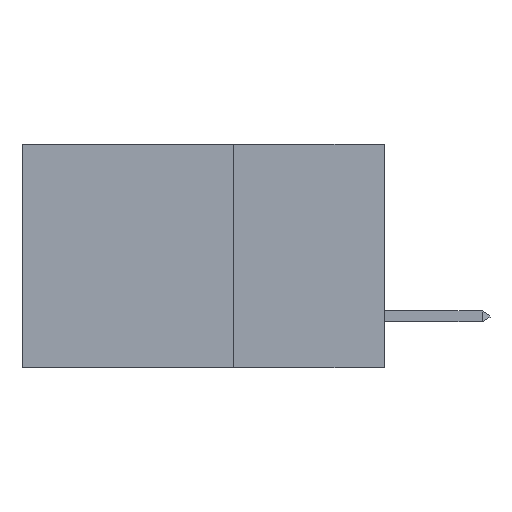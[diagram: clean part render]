
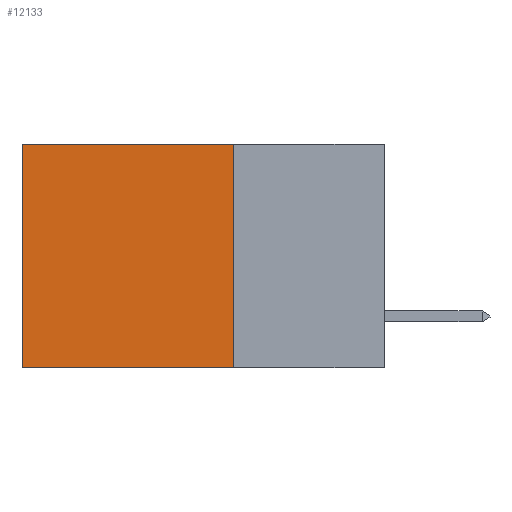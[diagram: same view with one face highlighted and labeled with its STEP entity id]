
A CAD part, left-side view. The second image highlights one B-rep face of the part: STEP entity #12133.
In plain terms, the highlighted planar face has unit normal (-1, 0, 0).
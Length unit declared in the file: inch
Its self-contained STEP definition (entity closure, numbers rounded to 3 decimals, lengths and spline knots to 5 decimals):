
#1130 = PLANE ( 'NONE',  #3478 ) ;
#1737 = DIRECTION ( 'NONE',  ( 0., 0., -1. ) ) ;
#3478 = AXIS2_PLACEMENT_3D ( 'NONE', #5786, #21544, #8066 ) ;
#3719 = EDGE_CURVE ( 'NONE', #9236, #6480, #10938, .T. ) ;
#4423 = LINE ( 'NONE', #21610, #21736 ) ;
#4626 = CARTESIAN_POINT ( 'NONE',  ( 0.2875, 0.25, 0. ) ) ;
#4700 = CARTESIAN_POINT ( 'NONE',  ( 0.2875, 0.25, 0. ) ) ;
#4757 = LINE ( 'NONE', #17261, #27944 ) ;
#4867 = VECTOR ( 'NONE', #27207, 39.37008 ) ;
#5786 = CARTESIAN_POINT ( 'NONE',  ( 0.2875, 0.25, 0. ) ) ;
#6480 = VERTEX_POINT ( 'NONE', #24880 ) ;
#8066 = DIRECTION ( 'NONE',  ( 0., 0., -1. ) ) ;
#8244 = ORIENTED_EDGE ( 'NONE', *, *, #28009, .T. ) ;
#9236 = VERTEX_POINT ( 'NONE', #4626 ) ;
#10371 = LINE ( 'NONE', #13140, #27513 ) ;
#10417 = DIRECTION ( 'NONE',  ( 0., 0., -1. ) ) ;
#10938 = LINE ( 'NONE', #4700, #4867 ) ;
#12133 = ADVANCED_FACE ( 'NONE', ( #21434 ), #1130, .F. ) ;
#12777 = EDGE_CURVE ( 'NONE', #9236, #13896, #4423, .T. ) ;
#13140 = CARTESIAN_POINT ( 'NONE',  ( 0.2875, 0.6, 0. ) ) ;
#13896 = VERTEX_POINT ( 'NONE', #25544 ) ;
#17261 = CARTESIAN_POINT ( 'NONE',  ( 0.2875, 0.25, -0.37 ) ) ;
#17993 = CARTESIAN_POINT ( 'NONE',  ( 0.2875, 0.6, -0.37 ) ) ;
#19038 = EDGE_CURVE ( 'NONE', #13896, #27482, #4757, .T. ) ;
#19493 = DIRECTION ( 'NONE',  ( 0., 1., 0. ) ) ;
#20326 = ORIENTED_EDGE ( 'NONE', *, *, #12777, .F. ) ;
#21434 = FACE_OUTER_BOUND ( 'NONE', #28768, .T. ) ;
#21544 = DIRECTION ( 'NONE',  ( 1., 0., 0. ) ) ;
#21610 = CARTESIAN_POINT ( 'NONE',  ( 0.2875, 0.25, 0. ) ) ;
#21736 = VECTOR ( 'NONE', #10417, 39.37008 ) ;
#24880 = CARTESIAN_POINT ( 'NONE',  ( 0.2875, 0.6, 0. ) ) ;
#25544 = CARTESIAN_POINT ( 'NONE',  ( 0.2875, 0.25, -0.37 ) ) ;
#27074 = ORIENTED_EDGE ( 'NONE', *, *, #19038, .F. ) ;
#27207 = DIRECTION ( 'NONE',  ( 0., 1., 0. ) ) ;
#27482 = VERTEX_POINT ( 'NONE', #17993 ) ;
#27513 = VECTOR ( 'NONE', #1737, 39.37008 ) ;
#27944 = VECTOR ( 'NONE', #19493, 39.37008 ) ;
#28009 = EDGE_CURVE ( 'NONE', #6480, #27482, #10371, .T. ) ;
#28654 = ORIENTED_EDGE ( 'NONE', *, *, #3719, .T. ) ;
#28768 = EDGE_LOOP ( 'NONE', ( #8244, #27074, #20326, #28654 ) ) ;
